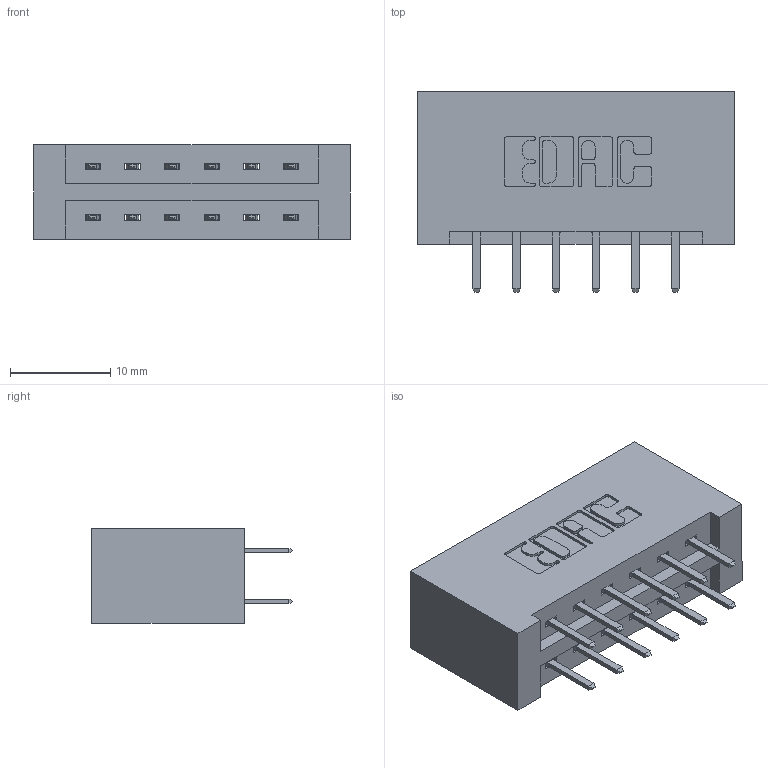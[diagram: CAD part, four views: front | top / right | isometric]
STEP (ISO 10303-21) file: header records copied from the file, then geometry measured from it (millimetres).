
FILE_DESCRIPTION (( 'STEP AP203' ), '1' );
FILE_NAME ('337-012-520-201.STEP', '2018-08-04T02:36:57', ( '' ), ( '' ), 'SwSTEP 2.0', 'SolidWorks 2016', '' );
FILE_SCHEMA (( 'CONFIG_CONTROL_DESIGN' ));
Length unit declared in the file: inch
Products named in the file (3): 337 Part_No Mounting Lugs; 345-292-001_345-293-120; 337-012-520-201
Assembly tree (13 placements, depth 2):
  337-012-520-201
    337 Part_No Mounting Lugs
    345-292-001_345-293-120  x12
Bounding box: 31.65 x 20.02 x 9.4 mm (x, y, z)
Volume: 3611.6 mm3; surface area: 3774.3 mm2
Topology: 13 solids, 13 shells, 802 faces, 2315 edges, 1510 vertices
Faces by surface type: plane 546, cylinder 256
Entity records: 9145 total; most frequent: CARTESIAN_POINT 1582, ORIENTED_EDGE 1506, DIRECTION 1393, EDGE_CURVE 753, LINE 629, VECTOR 629, VERTEX_POINT 498, AXIS2_PLACEMENT_3D 382
